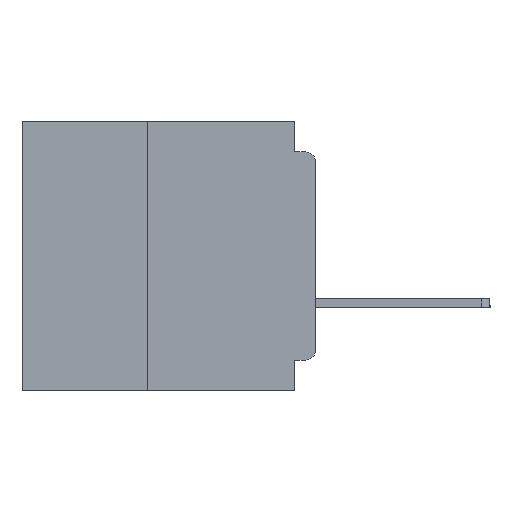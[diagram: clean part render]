
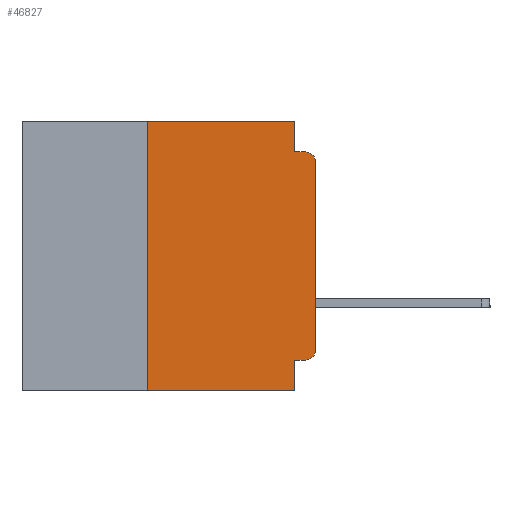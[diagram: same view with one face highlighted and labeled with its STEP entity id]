
A CAD part, left-side view. The second image highlights one B-rep face of the part: STEP entity #46827.
In plain terms, the highlighted planar face has unit normal (-1, 0, 0).
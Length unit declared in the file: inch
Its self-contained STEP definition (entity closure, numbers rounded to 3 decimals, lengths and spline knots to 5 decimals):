
#296 = CARTESIAN_POINT ( 'NONE',  ( 0., 0., -0.355 ) ) ;
#440 = DIRECTION ( 'NONE',  ( 0., 1., 0. ) ) ;
#469 = DIRECTION ( 'NONE',  ( 0., 0., -1. ) ) ;
#507 = LINE ( 'NONE', #12094, #26274 ) ;
#759 = VERTEX_POINT ( 'NONE', #20426 ) ;
#976 = CARTESIAN_POINT ( 'NONE',  ( 0., 0.015, -0.355 ) ) ;
#1792 = EDGE_CURVE ( 'NONE', #27884, #6368, #44636, .T. ) ;
#2023 = EDGE_CURVE ( 'NONE', #759, #38884, #24664, .T. ) ;
#2808 = LINE ( 'NONE', #23501, #10209 ) ;
#3256 = ORIENTED_EDGE ( 'NONE', *, *, #39594, .F. ) ;
#3302 = EDGE_CURVE ( 'NONE', #14854, #38884, #34328, .T. ) ;
#3954 = DIRECTION ( 'NONE',  ( 0., -1., 0. ) ) ;
#4048 = ORIENTED_EDGE ( 'NONE', *, *, #27671, .T. ) ;
#4739 = AXIS2_PLACEMENT_3D ( 'NONE', #7618, #22346, #469 ) ;
#5104 = CARTESIAN_POINT ( 'NONE',  ( 0., 0., -0.045 ) ) ;
#5407 = LINE ( 'NONE', #296, #23781 ) ;
#5815 = ORIENTED_EDGE ( 'NONE', *, *, #43733, .F. ) ;
#6210 = CARTESIAN_POINT ( 'NONE',  ( 0., 0.031, -0.4 ) ) ;
#6368 = VERTEX_POINT ( 'NONE', #10323 ) ;
#7618 = CARTESIAN_POINT ( 'NONE',  ( 0., 0.437, 0. ) ) ;
#8371 = ORIENTED_EDGE ( 'NONE', *, *, #8703, .F. ) ;
#8703 = EDGE_CURVE ( 'NONE', #22380, #43460, #13727, .T. ) ;
#9322 = DIRECTION ( 'NONE',  ( 0., 0., -1. ) ) ;
#9765 = DIRECTION ( 'NONE',  ( 0., 0., 1. ) ) ;
#10209 = VECTOR ( 'NONE', #23337, 39.37008 ) ;
#10323 = CARTESIAN_POINT ( 'NONE',  ( 0., 0.25, 0. ) ) ;
#11263 = PLANE ( 'NONE',  #4739 ) ;
#11273 = CARTESIAN_POINT ( 'NONE',  ( 0., 0.015, -0.06 ) ) ;
#12094 = CARTESIAN_POINT ( 'NONE',  ( 0., 0.031, 0. ) ) ;
#13026 = VERTEX_POINT ( 'NONE', #22649 ) ;
#13727 = LINE ( 'NONE', #34985, #23471 ) ;
#13763 = ORIENTED_EDGE ( 'NONE', *, *, #1792, .F. ) ;
#14854 = VERTEX_POINT ( 'NONE', #33361 ) ;
#14864 = VECTOR ( 'NONE', #3954, 39.37008 ) ;
#14959 = AXIS2_PLACEMENT_3D ( 'NONE', #11273, #15655, #15602 ) ;
#15175 = LINE ( 'NONE', #28054, #46664 ) ;
#15602 = DIRECTION ( 'NONE',  ( 0., 0., -1. ) ) ;
#15655 = DIRECTION ( 'NONE',  ( -1., 0., 0. ) ) ;
#16577 = ORIENTED_EDGE ( 'NONE', *, *, #46399, .F. ) ;
#18779 = FACE_OUTER_BOUND ( 'NONE', #37579, .T. ) ;
#18967 = CARTESIAN_POINT ( 'NONE',  ( 0., 0.015, -0.34 ) ) ;
#19022 = CIRCLE ( 'NONE', #29116, 0.015 ) ;
#20426 = CARTESIAN_POINT ( 'NONE',  ( 0., 0.031, -0.045 ) ) ;
#20919 = ORIENTED_EDGE ( 'NONE', *, *, #24184, .T. ) ;
#22122 = CARTESIAN_POINT ( 'NONE',  ( 0., 0.031, -0.355 ) ) ;
#22346 = DIRECTION ( 'NONE',  ( 1., 0., 0. ) ) ;
#22380 = VERTEX_POINT ( 'NONE', #22122 ) ;
#22649 = CARTESIAN_POINT ( 'NONE',  ( 0., 0., -0.34 ) ) ;
#22654 = DIRECTION ( 'NONE',  ( 0., 0., -1. ) ) ;
#23337 = DIRECTION ( 'NONE',  ( 0., -1., 0. ) ) ;
#23471 = VECTOR ( 'NONE', #9322, 39.37008 ) ;
#23501 = CARTESIAN_POINT ( 'NONE',  ( 0., 0.437, 0. ) ) ;
#23781 = VECTOR ( 'NONE', #440, 39.37008 ) ;
#24184 = EDGE_CURVE ( 'NONE', #28357, #13026, #19022, .T. ) ;
#24664 = LINE ( 'NONE', #5104, #14864 ) ;
#25140 = CARTESIAN_POINT ( 'NONE',  ( 0., 0.015, -0.045 ) ) ;
#26274 = VECTOR ( 'NONE', #37970, 39.37008 ) ;
#26404 = VECTOR ( 'NONE', #29667, 39.37008 ) ;
#27582 = CARTESIAN_POINT ( 'NONE',  ( 0., 0.25, -0.4 ) ) ;
#27671 = EDGE_CURVE ( 'NONE', #27884, #43460, #43595, .T. ) ;
#27884 = VERTEX_POINT ( 'NONE', #27582 ) ;
#28054 = CARTESIAN_POINT ( 'NONE',  ( 0., 0., 0. ) ) ;
#28357 = VERTEX_POINT ( 'NONE', #976 ) ;
#29116 = AXIS2_PLACEMENT_3D ( 'NONE', #18967, #44538, #22654 ) ;
#29667 = DIRECTION ( 'NONE',  ( 0., 0., 1. ) ) ;
#29743 = ORIENTED_EDGE ( 'NONE', *, *, #32438, .T. ) ;
#29873 = CARTESIAN_POINT ( 'NONE',  ( 0., 0.25, -0.4 ) ) ;
#29997 = CARTESIAN_POINT ( 'NONE',  ( 0., 0.437, -0.4 ) ) ;
#32438 = EDGE_CURVE ( 'NONE', #13026, #14854, #15175, .T. ) ;
#33361 = CARTESIAN_POINT ( 'NONE',  ( 0., 0., -0.06 ) ) ;
#33659 = DIRECTION ( 'NONE',  ( 0., -1., 0. ) ) ;
#33660 = ORIENTED_EDGE ( 'NONE', *, *, #3302, .T. ) ;
#33814 = VECTOR ( 'NONE', #33659, 39.37008 ) ;
#33924 = ORIENTED_EDGE ( 'NONE', *, *, #2023, .F. ) ;
#34328 = CIRCLE ( 'NONE', #14959, 0.015 ) ;
#34985 = CARTESIAN_POINT ( 'NONE',  ( 0., 0.031, -0.4 ) ) ;
#37579 = EDGE_LOOP ( 'NONE', ( #29743, #33660, #33924, #5815, #16577, #13763, #4048, #8371, #3256, #20919 ) ) ;
#37970 = DIRECTION ( 'NONE',  ( 0., 0., -1. ) ) ;
#38884 = VERTEX_POINT ( 'NONE', #25140 ) ;
#39594 = EDGE_CURVE ( 'NONE', #28357, #22380, #5407, .T. ) ;
#40889 = VERTEX_POINT ( 'NONE', #41691 ) ;
#41691 = CARTESIAN_POINT ( 'NONE',  ( 0., 0.031, 0. ) ) ;
#43460 = VERTEX_POINT ( 'NONE', #6210 ) ;
#43595 = LINE ( 'NONE', #29997, #33814 ) ;
#43733 = EDGE_CURVE ( 'NONE', #40889, #759, #507, .T. ) ;
#44538 = DIRECTION ( 'NONE',  ( -1., 0., 0. ) ) ;
#44636 = LINE ( 'NONE', #29873, #26404 ) ;
#46399 = EDGE_CURVE ( 'NONE', #6368, #40889, #2808, .T. ) ;
#46664 = VECTOR ( 'NONE', #9765, 39.37008 ) ;
#46827 = ADVANCED_FACE ( 'NONE', ( #18779 ), #11263, .F. ) ;
